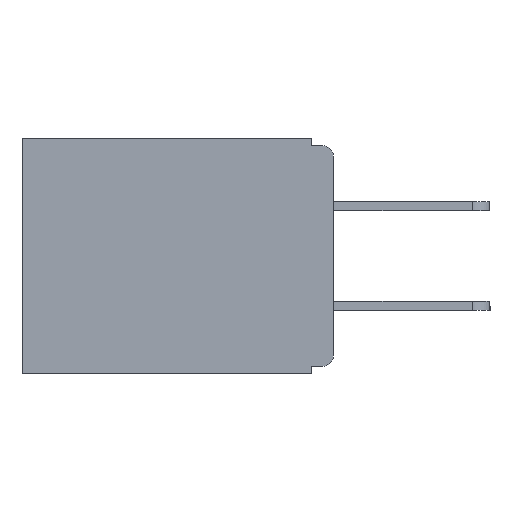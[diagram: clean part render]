
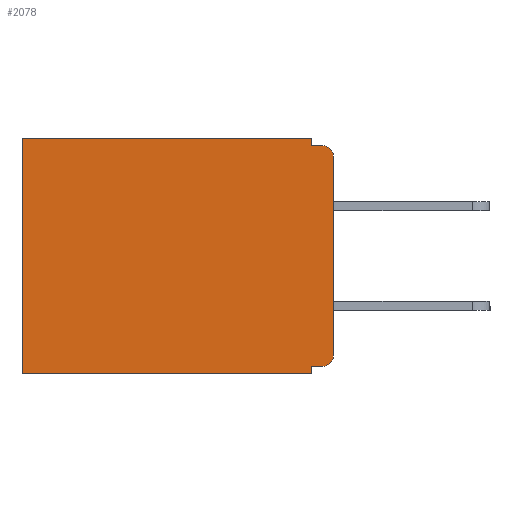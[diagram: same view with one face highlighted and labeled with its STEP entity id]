
A CAD part, left-side view. The second image highlights one B-rep face of the part: STEP entity #2078.
In plain terms, the highlighted planar face has unit normal (-1, 0, 0).
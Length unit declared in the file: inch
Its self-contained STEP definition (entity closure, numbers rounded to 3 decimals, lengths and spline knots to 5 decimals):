
#160 = DIRECTION ( 'NONE',  ( 0., 0., -1. ) ) ;
#612 = EDGE_CURVE ( 'NONE', #2094, #13691, #11935, .T. ) ;
#879 = EDGE_CURVE ( 'NONE', #17248, #1480, #15525, .T. ) ;
#949 = VECTOR ( 'NONE', #9795, 39.37008 ) ;
#1480 = VERTEX_POINT ( 'NONE', #15881 ) ;
#1482 = LINE ( 'NONE', #18441, #949 ) ;
#1524 = LINE ( 'NONE', #8796, #9249 ) ;
#1771 = ORIENTED_EDGE ( 'NONE', *, *, #14866, .T. ) ;
#1825 = ORIENTED_EDGE ( 'NONE', *, *, #879, .F. ) ;
#2078 = ADVANCED_FACE ( 'NONE', ( #12364 ), #2654, .F. ) ;
#2094 = VERTEX_POINT ( 'NONE', #13842 ) ;
#2199 = EDGE_CURVE ( 'NONE', #17041, #17248, #17729, .T. ) ;
#2294 = VERTEX_POINT ( 'NONE', #9896 ) ;
#2306 = VECTOR ( 'NONE', #18919, 39.37008 ) ;
#2654 = PLANE ( 'NONE',  #12948 ) ;
#2883 = ORIENTED_EDGE ( 'NONE', *, *, #12738, .T. ) ;
#3094 = ORIENTED_EDGE ( 'NONE', *, *, #5000, .F. ) ;
#3172 = VECTOR ( 'NONE', #4986, 39.37008 ) ;
#4431 = DIRECTION ( 'NONE',  ( -1., 0., 0. ) ) ;
#4986 = DIRECTION ( 'NONE',  ( 0., 0., -1. ) ) ;
#5000 = EDGE_CURVE ( 'NONE', #14439, #14715, #9970, .T. ) ;
#5645 = CIRCLE ( 'NONE', #12666, 0.015 ) ;
#5692 = ORIENTED_EDGE ( 'NONE', *, *, #612, .F. ) ;
#6000 = CARTESIAN_POINT ( 'NONE',  ( 0.3, 0., -0.33 ) ) ;
#6022 = CIRCLE ( 'NONE', #18603, 0.015 ) ;
#6255 = CARTESIAN_POINT ( 'NONE',  ( 0.3, 0., -0.33 ) ) ;
#6770 = DIRECTION ( 'NONE',  ( -1., 0., 0. ) ) ;
#7140 = CARTESIAN_POINT ( 'NONE',  ( 0.3, 0., -0.025 ) ) ;
#7691 = CARTESIAN_POINT ( 'NONE',  ( 0.3, 0.031, 0. ) ) ;
#7893 = ORIENTED_EDGE ( 'NONE', *, *, #11154, .T. ) ;
#7941 = ORIENTED_EDGE ( 'NONE', *, *, #17430, .F. ) ;
#7994 = ORIENTED_EDGE ( 'NONE', *, *, #13326, .F. ) ;
#8019 = VECTOR ( 'NONE', #11150, 39.37008 ) ;
#8796 = CARTESIAN_POINT ( 'NONE',  ( 0.3, 0., -0.01 ) ) ;
#9249 = VECTOR ( 'NONE', #11842, 39.37008 ) ;
#9795 = DIRECTION ( 'NONE',  ( 0., 1., 0. ) ) ;
#9896 = CARTESIAN_POINT ( 'NONE',  ( 0.3, 0.437, 0. ) ) ;
#9970 = LINE ( 'NONE', #6255, #2306 ) ;
#10439 = ORIENTED_EDGE ( 'NONE', *, *, #16585, .T. ) ;
#10498 = VECTOR ( 'NONE', #12131, 39.37008 ) ;
#10910 = EDGE_LOOP ( 'NONE', ( #3094, #10439, #7994, #5692, #1771, #7893, #7941, #1825, #17176, #2883 ) ) ;
#10934 = VERTEX_POINT ( 'NONE', #17090 ) ;
#10952 = CARTESIAN_POINT ( 'NONE',  ( 0.3, 0., -0.305 ) ) ;
#11150 = DIRECTION ( 'NONE',  ( 0., 0., -1. ) ) ;
#11154 = EDGE_CURVE ( 'NONE', #2294, #11222, #17513, .T. ) ;
#11222 = VERTEX_POINT ( 'NONE', #14119 ) ;
#11842 = DIRECTION ( 'NONE',  ( 0., -1., 0. ) ) ;
#11935 = LINE ( 'NONE', #7691, #8019 ) ;
#11980 = DIRECTION ( 'NONE',  ( 0., 1., 0. ) ) ;
#12131 = DIRECTION ( 'NONE',  ( 0., 1., 0. ) ) ;
#12364 = FACE_OUTER_BOUND ( 'NONE', #10910, .T. ) ;
#12666 = AXIS2_PLACEMENT_3D ( 'NONE', #15530, #6770, #16970 ) ;
#12738 = EDGE_CURVE ( 'NONE', #17041, #14715, #6022, .T. ) ;
#12948 = AXIS2_PLACEMENT_3D ( 'NONE', #17026, #18783, #160 ) ;
#13125 = CARTESIAN_POINT ( 'NONE',  ( 0.3, 0., -0.32 ) ) ;
#13239 = VECTOR ( 'NONE', #15054, 39.37008 ) ;
#13326 = EDGE_CURVE ( 'NONE', #13691, #10934, #1524, .T. ) ;
#13364 = CARTESIAN_POINT ( 'NONE',  ( 0.3, 0.015, -0.305 ) ) ;
#13687 = CARTESIAN_POINT ( 'NONE',  ( 0.3, 0.031, -0.33 ) ) ;
#13691 = VERTEX_POINT ( 'NONE', #16989 ) ;
#13842 = CARTESIAN_POINT ( 'NONE',  ( 0.3, 0.031, 0. ) ) ;
#13977 = CARTESIAN_POINT ( 'NONE',  ( 0.3, 0.015, -0.32 ) ) ;
#14119 = CARTESIAN_POINT ( 'NONE',  ( 0.3, 0.437, -0.33 ) ) ;
#14439 = VERTEX_POINT ( 'NONE', #7140 ) ;
#14662 = VECTOR ( 'NONE', #11980, 39.37008 ) ;
#14715 = VERTEX_POINT ( 'NONE', #10952 ) ;
#14805 = DIRECTION ( 'NONE',  ( 0., 0., -1. ) ) ;
#14866 = EDGE_CURVE ( 'NONE', #2094, #2294, #1482, .T. ) ;
#14994 = CARTESIAN_POINT ( 'NONE',  ( 0.3, 0.437, -0.33 ) ) ;
#15054 = DIRECTION ( 'NONE',  ( 0., 0., -1. ) ) ;
#15133 = LINE ( 'NONE', #6000, #14662 ) ;
#15525 = LINE ( 'NONE', #13687, #3172 ) ;
#15530 = CARTESIAN_POINT ( 'NONE',  ( 0.3, 0.015, -0.025 ) ) ;
#15865 = CARTESIAN_POINT ( 'NONE',  ( 0.3, 0.031, -0.32 ) ) ;
#15881 = CARTESIAN_POINT ( 'NONE',  ( 0.3, 0.031, -0.33 ) ) ;
#16585 = EDGE_CURVE ( 'NONE', #14439, #10934, #5645, .T. ) ;
#16970 = DIRECTION ( 'NONE',  ( 0., 0., -1. ) ) ;
#16989 = CARTESIAN_POINT ( 'NONE',  ( 0.3, 0.031, -0.01 ) ) ;
#17026 = CARTESIAN_POINT ( 'NONE',  ( 0.3, 0., -0.33 ) ) ;
#17041 = VERTEX_POINT ( 'NONE', #13977 ) ;
#17090 = CARTESIAN_POINT ( 'NONE',  ( 0.3, 0.015, -0.01 ) ) ;
#17176 = ORIENTED_EDGE ( 'NONE', *, *, #2199, .F. ) ;
#17248 = VERTEX_POINT ( 'NONE', #15865 ) ;
#17430 = EDGE_CURVE ( 'NONE', #1480, #11222, #15133, .T. ) ;
#17513 = LINE ( 'NONE', #14994, #13239 ) ;
#17729 = LINE ( 'NONE', #13125, #10498 ) ;
#18441 = CARTESIAN_POINT ( 'NONE',  ( 0.3, 0., 0. ) ) ;
#18603 = AXIS2_PLACEMENT_3D ( 'NONE', #13364, #4431, #14805 ) ;
#18783 = DIRECTION ( 'NONE',  ( 1., 0., 0. ) ) ;
#18919 = DIRECTION ( 'NONE',  ( 0., 0., -1. ) ) ;
